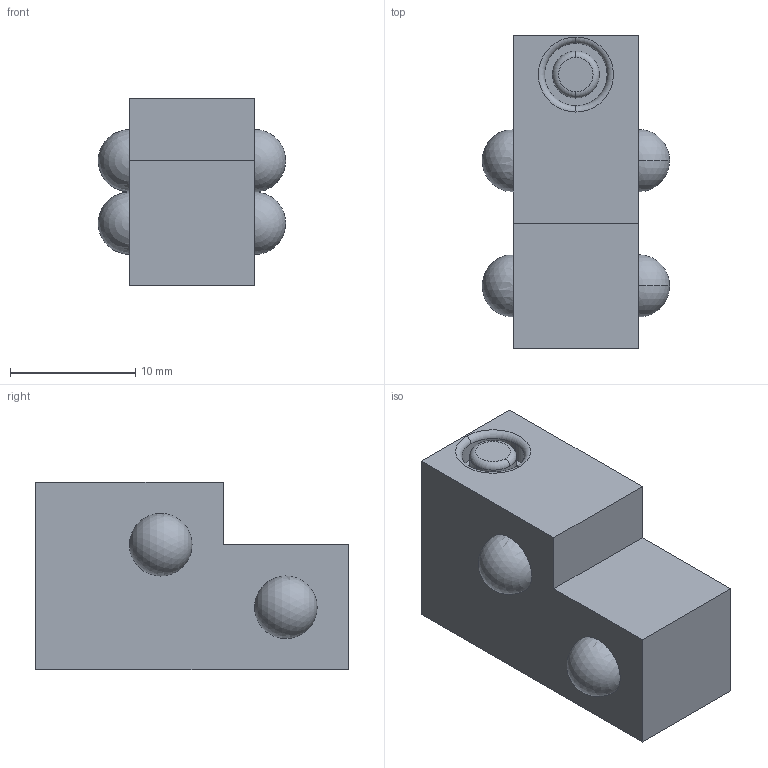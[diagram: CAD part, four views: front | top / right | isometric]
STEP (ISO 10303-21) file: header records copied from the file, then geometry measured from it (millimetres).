
FILE_DESCRIPTION (( 'STEP AP214' ), '1' );
FILE_NAME ('Hinge_Cover.step', '2013-11-06T14:31:09', ( 'elpi' ), ( '' ), 'SwSTEP 2.0', 'SolidWorks 2013', '' );
FILE_SCHEMA (( 'AUTOMOTIVE_DESIGN' ));
Length unit declared in the file: millimetre
Products named in the file (1): Hinge_Cover
Bounding box: 14.98 x 25 x 15 mm (x, y, z)
Volume: 3362.2 mm3; surface area: 1577.6 mm2
Topology: 1 solids, 1 shells, 24 faces, 68 edges, 44 vertices
Faces by surface type: plane 10, sphere 6, torus 4, cylinder 4
Entity records: 712 total; most frequent: DIRECTION 132, CARTESIAN_POINT 113, ORIENTED_EDGE 104, AXIS2_PLACEMENT_3D 55, EDGE_CURVE 52, VERTEX_POINT 36, CIRCLE 30, EDGE_LOOP 30
